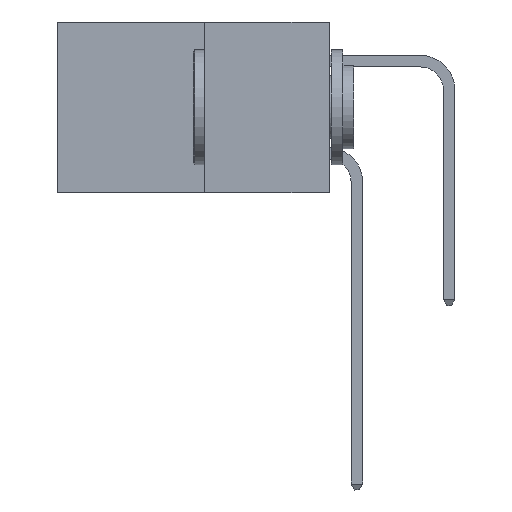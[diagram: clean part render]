
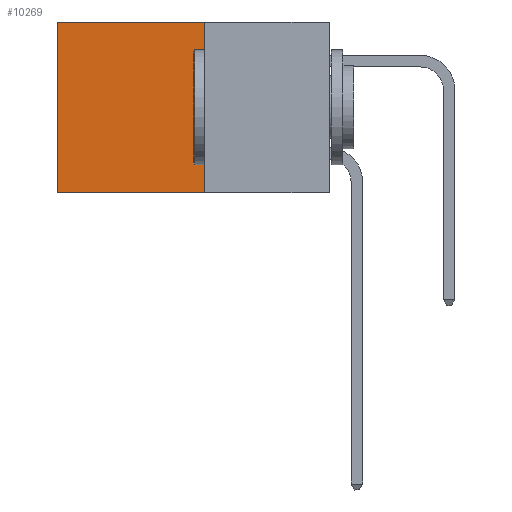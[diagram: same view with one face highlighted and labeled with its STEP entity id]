
A CAD part, left-side view. The second image highlights one B-rep face of the part: STEP entity #10269.
In plain terms, the highlighted planar face has unit normal (-1, 0, 0).
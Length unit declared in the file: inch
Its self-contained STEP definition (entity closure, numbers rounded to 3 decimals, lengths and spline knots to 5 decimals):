
#823 = VERTEX_POINT ( 'NONE', #8973 ) ;
#838 = EDGE_CURVE ( 'NONE', #5374, #823, #8061, .T. ) ;
#1413 = EDGE_CURVE ( 'NONE', #10120, #823, #4699, .T. ) ;
#1416 = EDGE_CURVE ( 'NONE', #1449, #5374, #4405, .T. ) ;
#1448 = LINE ( 'NONE', #3745, #4081 ) ;
#1449 = VERTEX_POINT ( 'NONE', #9150 ) ;
#1493 = VECTOR ( 'NONE', #11029, 39.37008 ) ;
#1629 = CARTESIAN_POINT ( 'NONE',  ( 0.277, 0.59, 0. ) ) ;
#2041 = EDGE_CURVE ( 'NONE', #1449, #10120, #1448, .T. ) ;
#2399 = DIRECTION ( 'NONE',  ( 1., 0., 0. ) ) ;
#2941 = EDGE_LOOP ( 'NONE', ( #3789, #5722, #9153, #3823 ) ) ;
#3411 = DIRECTION ( 'NONE',  ( 0., 0., -1. ) ) ;
#3445 = CARTESIAN_POINT ( 'NONE',  ( 0.277, 0.27, -0.37 ) ) ;
#3745 = CARTESIAN_POINT ( 'NONE',  ( 0.277, 0.27, -0.37 ) ) ;
#3789 = ORIENTED_EDGE ( 'NONE', *, *, #838, .T. ) ;
#3823 = ORIENTED_EDGE ( 'NONE', *, *, #1416, .T. ) ;
#4081 = VECTOR ( 'NONE', #3411, 39.37008 ) ;
#4360 = CARTESIAN_POINT ( 'NONE',  ( 0.277, 0.27, -0.37 ) ) ;
#4405 = LINE ( 'NONE', #11032, #1493 ) ;
#4699 = LINE ( 'NONE', #11725, #9014 ) ;
#5374 = VERTEX_POINT ( 'NONE', #1629 ) ;
#5375 = PLANE ( 'NONE',  #9524 ) ;
#5722 = ORIENTED_EDGE ( 'NONE', *, *, #1413, .F. ) ;
#6152 = VECTOR ( 'NONE', #7102, 39.37008 ) ;
#7102 = DIRECTION ( 'NONE',  ( 0., 0., -1. ) ) ;
#8061 = LINE ( 'NONE', #9846, #6152 ) ;
#8789 = DIRECTION ( 'NONE',  ( 0., 0., -1. ) ) ;
#8973 = CARTESIAN_POINT ( 'NONE',  ( 0.277, 0.59, -0.37 ) ) ;
#9014 = VECTOR ( 'NONE', #11553, 39.37008 ) ;
#9150 = CARTESIAN_POINT ( 'NONE',  ( 0.277, 0.27, 0. ) ) ;
#9153 = ORIENTED_EDGE ( 'NONE', *, *, #2041, .F. ) ;
#9524 = AXIS2_PLACEMENT_3D ( 'NONE', #3445, #2399, #8789 ) ;
#9846 = CARTESIAN_POINT ( 'NONE',  ( 0.277, 0.59, -0.37 ) ) ;
#10120 = VERTEX_POINT ( 'NONE', #4360 ) ;
#10269 = ADVANCED_FACE ( 'NONE', ( #11647 ), #5375, .F. ) ;
#11029 = DIRECTION ( 'NONE',  ( 0., 1., 0. ) ) ;
#11032 = CARTESIAN_POINT ( 'NONE',  ( 0.277, 0.27, 0. ) ) ;
#11553 = DIRECTION ( 'NONE',  ( 0., 1., 0. ) ) ;
#11647 = FACE_OUTER_BOUND ( 'NONE', #2941, .T. ) ;
#11725 = CARTESIAN_POINT ( 'NONE',  ( 0.277, 0.27, -0.37 ) ) ;
